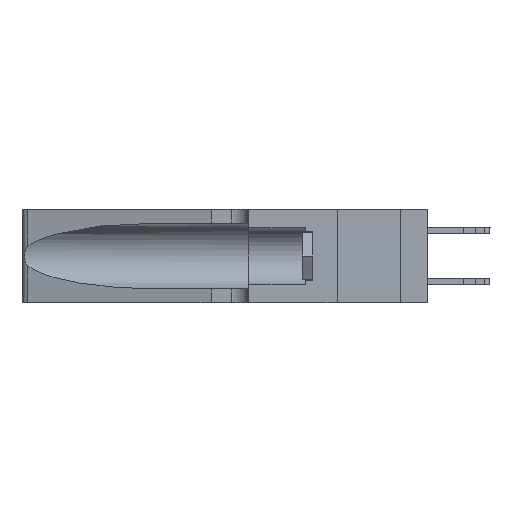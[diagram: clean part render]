
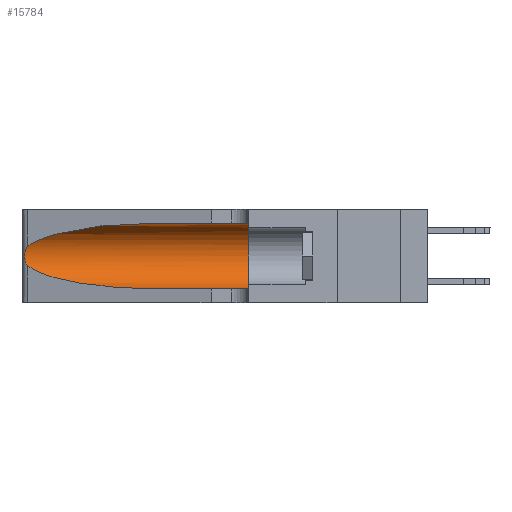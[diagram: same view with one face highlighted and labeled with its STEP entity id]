
A CAD part, left-side view. The second image highlights one B-rep face of the part: STEP entity #15784.
In plain terms, the highlighted cylindrical face has radius 3.308 mm (diameter 6.617 mm), a partial arc.
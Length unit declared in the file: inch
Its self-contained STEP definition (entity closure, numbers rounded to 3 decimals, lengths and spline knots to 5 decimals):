
#858 = ORIENTED_EDGE ( 'NONE', *, *, #13030, .T. ) ;
#903 = VERTEX_POINT ( 'NONE', #11891 ) ;
#905 = CARTESIAN_POINT ( 'NONE',  ( 0.25854, 1.2359, 0.20912 ) ) ;
#975 = CARTESIAN_POINT ( 'NONE',  ( 0.26075, 1.23896, 0.19203 ) ) ;
#1448 = VECTOR ( 'NONE', #9636, 39.37008 ) ;
#2364 = CARTESIAN_POINT ( 'NONE',  ( 0.18966, 0.96281, 0.31525 ) ) ;
#2438 = CARTESIAN_POINT ( 'NONE',  ( 0.2373, 1.15595, 0.08982 ) ) ;
#2457 = CARTESIAN_POINT ( 'NONE',  ( 0.25555, 1.22994, 0.2215 ) ) ;
#2613 = CARTESIAN_POINT ( 'NONE',  ( 0.25856, 1.23593, 0.16098 ) ) ;
#2679 = VERTEX_POINT ( 'NONE', #5601 ) ;
#3368 = EDGE_CURVE ( 'NONE', #903, #18011, #17594, .T. ) ;
#3483 = CARTESIAN_POINT ( 'NONE',  ( 0.1305, 1.61858, 0.05475 ) ) ;
#3636 = DIRECTION ( 'NONE',  ( 0., 0., -1. ) ) ;
#4119 = ORIENTED_EDGE ( 'NONE', *, *, #11340, .T. ) ;
#4131 = CARTESIAN_POINT ( 'NONE',  ( 0.25639, 1.23184, 0.21858 ) ) ;
#4289 = CARTESIAN_POINT ( 'NONE',  ( 0.25555, 1.22993, 0.14849 ) ) ;
#4642 = CARTESIAN_POINT ( 'NONE',  ( 0.2373, 1.15595, 0.28018 ) ) ;
#4995 = DIRECTION ( 'NONE',  ( 0., 0., 1. ) ) ;
#5291 = ORIENTED_EDGE ( 'NONE', *, *, #3368, .T. ) ;
#5297 = EDGE_CURVE ( 'NONE', #14451, #18404, #21139, .T. ) ;
#5554 = ORIENTED_EDGE ( 'NONE', *, *, #13953, .F. ) ;
#5601 = CARTESIAN_POINT ( 'NONE',  ( 0.1305, 0.35, 0.05475 ) ) ;
#5874 = CARTESIAN_POINT ( 'NONE',  ( 0.18966, 0.96281, 0.05475 ) ) ;
#5895 = CARTESIAN_POINT ( 'NONE',  ( 0.26018, 1.23835, 0.19895 ) ) ;
#6776 = CARTESIAN_POINT ( 'NONE',  ( 0.1305, 0.35, 0.31525 ) ) ;
#7669 = CARTESIAN_POINT ( 'NONE',  ( 0.26075, 1.23896, 0.178 ) ) ;
#7727 = ORIENTED_EDGE ( 'NONE', *, *, #5297, .T. ) ;
#7892 = CIRCLE ( 'NONE', #14786, 0.13025 ) ;
#8923 = DIRECTION ( 'NONE',  ( 0., -1., 0. ) ) ;
#9260 = CARTESIAN_POINT ( 'NONE',  ( 0.25787, 1.23484, 0.2124 ) ) ;
#9636 = DIRECTION ( 'NONE',  ( 0., -1., 0. ) ) ;
#10575 = DIRECTION ( 'NONE',  ( 0., 1., 0. ) ) ;
#10710 = FACE_OUTER_BOUND ( 'NONE', #14228, .T. ) ;
#10734 = CARTESIAN_POINT ( 'NONE',  ( 0.1305, 1.61858, 0.185 ) ) ;
#11133 = CARTESIAN_POINT ( 'NONE',  ( 0.26017, 1.23833, 0.17102 ) ) ;
#11340 = EDGE_CURVE ( 'NONE', #18011, #2679, #17865, .T. ) ;
#11891 = CARTESIAN_POINT ( 'NONE',  ( 0.25487, 1.22718, 0.14631 ) ) ;
#12227 = EDGE_CURVE ( 'NONE', #14451, #18976, #13018, .T. ) ;
#12488 = CARTESIAN_POINT ( 'NONE',  ( 0.25487, 1.22718, 0.22369 ) ) ;
#12753 = ORIENTED_EDGE ( 'NONE', *, *, #12227, .F. ) ;
#13018 = LINE ( 'NONE', #17989, #1448 ) ;
#13030 = EDGE_CURVE ( 'NONE', #18404, #903, #15291, .T. ) ;
#13953 = EDGE_CURVE ( 'NONE', #18976, #2679, #7892, .T. ) ;
#14185 = CYLINDRICAL_SURFACE ( 'NONE', #15663, 0.13025 ) ;
#14228 = EDGE_LOOP ( 'NONE', ( #7727, #858, #5291, #4119, #5554, #12753 ) ) ;
#14451 = VERTEX_POINT ( 'NONE', #22105 ) ;
#14786 = AXIS2_PLACEMENT_3D ( 'NONE', #15290, #10575, #4995 ) ;
#15290 = CARTESIAN_POINT ( 'NONE',  ( 0.1305, 0.35, 0.185 ) ) ;
#15291 = B_SPLINE_CURVE_WITH_KNOTS ( 'NONE', 3,
 ( #17911, #2457, #4131, #9260, #905, #5895, #975, #7669, #11133, #2613, #16366, #21344, #4289, #21191 ),
 .UNSPECIFIED., .F., .F.,
 ( 4, 2, 2, 2, 2, 2, 4 ),
 ( 0., 0.00027, 0.00053, 0.00107, 0.0016, 0.00187, 0.00214 ),
 .UNSPECIFIED. ) ;
#15582 = DIRECTION ( 'NONE',  ( 0., -1., 0. ) ) ;
#15663 = AXIS2_PLACEMENT_3D ( 'NONE', #10734, #8923, #3636 ) ;
#15784 = ADVANCED_FACE ( 'NONE', ( #10710 ), #14185, .F. ) ;
#16199 = CARTESIAN_POINT ( 'NONE',  ( 0.1305, 0.72297, 0.05475 ) ) ;
#16366 = CARTESIAN_POINT ( 'NONE',  ( 0.25789, 1.23486, 0.15765 ) ) ;
#17097 = VECTOR ( 'NONE', #15582, 39.37008 ) ;
#17594 =( BOUNDED_CURVE ( )  B_SPLINE_CURVE ( 3, ( #21249, #2438, #5874, #16199 ),
 .UNSPECIFIED., .F., .F. ) 
 B_SPLINE_CURVE_WITH_KNOTS ( ( 4, 4 ),
 ( 3.44316, 4.71239 ),
 .UNSPECIFIED. ) 
 CURVE ( )  GEOMETRIC_REPRESENTATION_ITEM ( )  RATIONAL_B_SPLINE_CURVE ( ( 1., 0.87, 0.87, 1. ) ) 
 REPRESENTATION_ITEM ( '' )  );
#17865 = LINE ( 'NONE', #3483, #17097 ) ;
#17911 = CARTESIAN_POINT ( 'NONE',  ( 0.25487, 1.22718, 0.22369 ) ) ;
#17989 = CARTESIAN_POINT ( 'NONE',  ( 0.1305, 1.61858, 0.31525 ) ) ;
#18011 = VERTEX_POINT ( 'NONE', #21692 ) ;
#18404 = VERTEX_POINT ( 'NONE', #12488 ) ;
#18976 = VERTEX_POINT ( 'NONE', #6776 ) ;
#19456 = CARTESIAN_POINT ( 'NONE',  ( 0.1305, 0.72297, 0.31525 ) ) ;
#20055 = CARTESIAN_POINT ( 'NONE',  ( 0.25487, 1.22718, 0.22369 ) ) ;
#21139 =( BOUNDED_CURVE ( )  B_SPLINE_CURVE ( 3, ( #19456, #2364, #4642, #20055 ),
 .UNSPECIFIED., .F., .T. ) 
 B_SPLINE_CURVE_WITH_KNOTS ( ( 4, 4 ),
 ( 1.5708, 2.84003 ),
 .UNSPECIFIED. ) 
 CURVE ( )  GEOMETRIC_REPRESENTATION_ITEM ( )  RATIONAL_B_SPLINE_CURVE ( ( 1., 0.87, 0.87, 1. ) ) 
 REPRESENTATION_ITEM ( '' )  );
#21191 = CARTESIAN_POINT ( 'NONE',  ( 0.25487, 1.22718, 0.14631 ) ) ;
#21249 = CARTESIAN_POINT ( 'NONE',  ( 0.25487, 1.22718, 0.14631 ) ) ;
#21344 = CARTESIAN_POINT ( 'NONE',  ( 0.25639, 1.23186, 0.15144 ) ) ;
#21692 = CARTESIAN_POINT ( 'NONE',  ( 0.1305, 0.72297, 0.05475 ) ) ;
#22105 = CARTESIAN_POINT ( 'NONE',  ( 0.1305, 0.72297, 0.31525 ) ) ;
